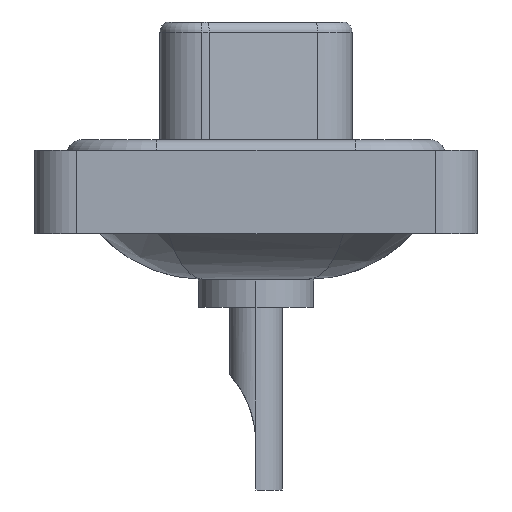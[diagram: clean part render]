
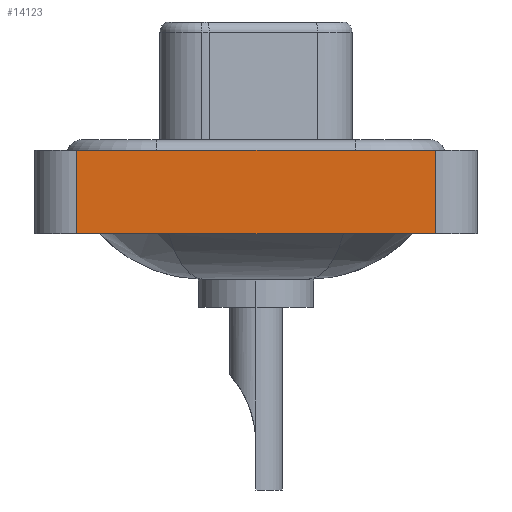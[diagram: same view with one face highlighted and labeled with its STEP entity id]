
A CAD part, left-side view. The second image highlights one B-rep face of the part: STEP entity #14123.
In plain terms, the highlighted planar face has unit normal (-1, 0, 0).
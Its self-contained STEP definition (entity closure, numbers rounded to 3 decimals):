
#32 = DIRECTION ( 'NONE',  ( 0., 0., 1. ) ) ;
#554 = LINE ( 'NONE', #14559, #16199 ) ;
#687 = ORIENTED_EDGE ( 'NONE', *, *, #13479, .T. ) ;
#1834 = PLANE ( 'NONE',  #11247 ) ;
#2522 = DIRECTION ( 'NONE',  ( 0., 0., 1. ) ) ;
#2620 = ORIENTED_EDGE ( 'NONE', *, *, #14313, .T. ) ;
#2709 = VERTEX_POINT ( 'NONE', #7096 ) ;
#2923 = DIRECTION ( 'NONE',  ( 0., -1., 0. ) ) ;
#3049 = VECTOR ( 'NONE', #2923, 1000. ) ;
#3211 = FACE_OUTER_BOUND ( 'NONE', #12386, .T. ) ;
#3401 = DIRECTION ( 'NONE',  ( 0., -1., 0. ) ) ;
#3925 = ORIENTED_EDGE ( 'NONE', *, *, #6525, .F. ) ;
#4252 = LINE ( 'NONE', #16887, #13195 ) ;
#4376 = ORIENTED_EDGE ( 'NONE', *, *, #4856, .F. ) ;
#4856 = EDGE_CURVE ( 'NONE', #15062, #16589, #554, .T. ) ;
#5616 = LINE ( 'NONE', #6636, #14718 ) ;
#5835 = CARTESIAN_POINT ( 'NONE',  ( -7.25, -8.55, -3.6 ) ) ;
#6043 = DIRECTION ( 'NONE',  ( 0., 0., 1. ) ) ;
#6525 = EDGE_CURVE ( 'NONE', #7008, #15062, #5616, .T. ) ;
#6636 = CARTESIAN_POINT ( 'NONE',  ( -7.25, 8.55, -3.6 ) ) ;
#7008 = VERTEX_POINT ( 'NONE', #15045 ) ;
#7096 = CARTESIAN_POINT ( 'NONE',  ( -7.25, -8.55, -3.6 ) ) ;
#7425 = CARTESIAN_POINT ( 'NONE',  ( -7.25, -8.55, -3.6 ) ) ;
#10464 = DIRECTION ( 'NONE',  ( -1., 0., 0. ) ) ;
#11247 = AXIS2_PLACEMENT_3D ( 'NONE', #7425, #10464, #6043 ) ;
#11952 = CARTESIAN_POINT ( 'NONE',  ( -7.25, 8.55, 0.4 ) ) ;
#12386 = EDGE_LOOP ( 'NONE', ( #687, #4376, #3925, #2620 ) ) ;
#13195 = VECTOR ( 'NONE', #32, 1000. ) ;
#13479 = EDGE_CURVE ( 'NONE', #2709, #16589, #4252, .T. ) ;
#13713 = CARTESIAN_POINT ( 'NONE',  ( -7.25, -8.55, 0.4 ) ) ;
#14123 = ADVANCED_FACE ( 'NONE', ( #3211 ), #1834, .T. ) ;
#14313 = EDGE_CURVE ( 'NONE', #7008, #2709, #17575, .T. ) ;
#14559 = CARTESIAN_POINT ( 'NONE',  ( -7.25, -8.55, 0.4 ) ) ;
#14718 = VECTOR ( 'NONE', #2522, 1000. ) ;
#15045 = CARTESIAN_POINT ( 'NONE',  ( -7.25, 8.55, -3.6 ) ) ;
#15062 = VERTEX_POINT ( 'NONE', #11952 ) ;
#16199 = VECTOR ( 'NONE', #3401, 1000. ) ;
#16589 = VERTEX_POINT ( 'NONE', #13713 ) ;
#16887 = CARTESIAN_POINT ( 'NONE',  ( -7.25, -8.55, -3.6 ) ) ;
#17575 = LINE ( 'NONE', #5835, #3049 ) ;
